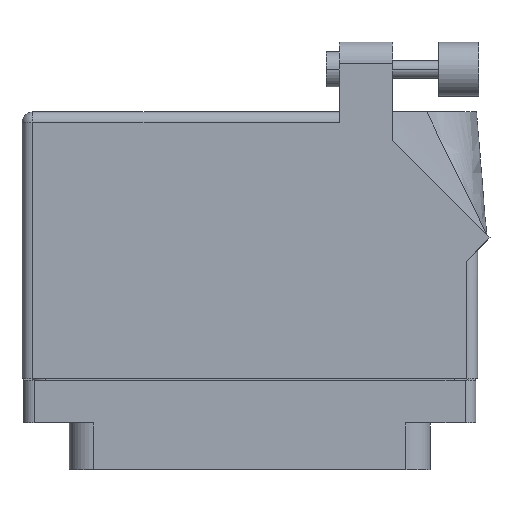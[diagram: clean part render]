
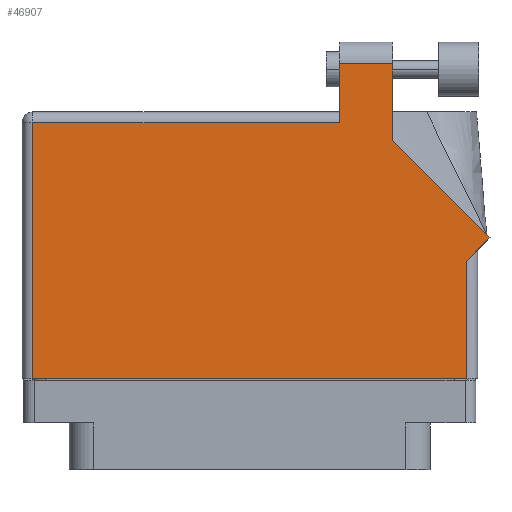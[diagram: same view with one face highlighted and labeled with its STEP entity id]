
A CAD part, front view. The second image highlights one B-rep face of the part: STEP entity #46907.
In plain terms, the highlighted face is planar.
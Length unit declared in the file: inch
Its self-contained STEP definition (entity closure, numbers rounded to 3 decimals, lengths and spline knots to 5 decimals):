
#619 = CARTESIAN_POINT ( 'NONE',  ( -1.306, 1.43, 0.455 ) ) ;
#1910 = ORIENTED_EDGE ( 'NONE', *, *, #14953, .T. ) ;
#3259 = EDGE_LOOP ( 'NONE', ( #28882, #19942, #36924, #26401, #10482, #31854, #46500, #20059, #1910 ) ) ;
#4054 = CARTESIAN_POINT ( 'NONE',  ( -1.306, 1.368, 0.455 ) ) ;
#4148 = FACE_OUTER_BOUND ( 'NONE', #3259, .T. ) ;
#4621 = LINE ( 'NONE', #43150, #7143 ) ;
#6073 = EDGE_CURVE ( 'NONE', #32057, #24403, #44355, .T. ) ;
#6397 = VECTOR ( 'NONE', #47494, 39.37008 ) ;
#7143 = VECTOR ( 'NONE', #19207, 39.37008 ) ;
#7683 = LINE ( 'NONE', #45672, #38993 ) ;
#8617 = VECTOR ( 'NONE', #9817, 39.37008 ) ;
#9040 = DIRECTION ( 'NONE',  ( 0., 0., -1. ) ) ;
#9306 = CARTESIAN_POINT ( 'NONE',  ( 1.37671, 0.70771, 0.455 ) ) ;
#9817 = DIRECTION ( 'NONE',  ( -0.707, 0.707, 0. ) ) ;
#10092 = VERTEX_POINT ( 'NONE', #9306 ) ;
#10482 = ORIENTED_EDGE ( 'NONE', *, *, #15534, .T. ) ;
#10491 = VECTOR ( 'NONE', #27867, 39.37008 ) ;
#10498 = VECTOR ( 'NONE', #36122, 39.37008 ) ;
#13023 = EDGE_CURVE ( 'NONE', #18668, #38605, #38357, .T. ) ;
#13599 = VERTEX_POINT ( 'NONE', #32196 ) ;
#14877 = LINE ( 'NONE', #44491, #10491 ) ;
#14953 = EDGE_CURVE ( 'NONE', #10092, #40217, #46825, .T. ) ;
#15534 = EDGE_CURVE ( 'NONE', #24403, #18668, #25461, .T. ) ;
#18668 = VERTEX_POINT ( 'NONE', #19791 ) ;
#19162 = VERTEX_POINT ( 'NONE', #19208 ) ;
#19207 = DIRECTION ( 'NONE',  ( 0., -1., 0. ) ) ;
#19208 = CARTESIAN_POINT ( 'NONE',  ( 0.513, 1.705, 0.455 ) ) ;
#19791 = CARTESIAN_POINT ( 'NONE',  ( -1.244, -0.1, 0.455 ) ) ;
#19942 = ORIENTED_EDGE ( 'NONE', *, *, #36647, .T. ) ;
#20059 = ORIENTED_EDGE ( 'NONE', *, *, #33033, .T. ) ;
#20361 = CARTESIAN_POINT ( 'NONE',  ( 0.82, 1.26442, 0.455 ) ) ;
#21722 = DIRECTION ( 'NONE',  ( 0.707, 0.707, 0. ) ) ;
#23365 = CARTESIAN_POINT ( 'NONE',  ( -1.306, -0.1, 0.455 ) ) ;
#24403 = VERTEX_POINT ( 'NONE', #25230 ) ;
#24527 = DIRECTION ( 'NONE',  ( 0., 1., 0. ) ) ;
#25230 = CARTESIAN_POINT ( 'NONE',  ( -1.244, 1.368, 0.455 ) ) ;
#25325 = EDGE_CURVE ( 'NONE', #38605, #26138, #28949, .T. ) ;
#25408 = CARTESIAN_POINT ( 'NONE',  ( 0.513, 1.368, 0.455 ) ) ;
#25461 = LINE ( 'NONE', #26735, #32988 ) ;
#26138 = VERTEX_POINT ( 'NONE', #33226 ) ;
#26401 = ORIENTED_EDGE ( 'NONE', *, *, #6073, .T. ) ;
#26735 = CARTESIAN_POINT ( 'NONE',  ( -1.244, -0.1, 0.455 ) ) ;
#27249 = EDGE_CURVE ( 'NONE', #40217, #13599, #30662, .T. ) ;
#27601 = DIRECTION ( 'NONE',  ( 0., 1., 0. ) ) ;
#27867 = DIRECTION ( 'NONE',  ( -1., 0., 0. ) ) ;
#28882 = ORIENTED_EDGE ( 'NONE', *, *, #27249, .T. ) ;
#28949 = LINE ( 'NONE', #51566, #40840 ) ;
#29771 = CARTESIAN_POINT ( 'NONE',  ( 1.37671, 0.70771, 0.455 ) ) ;
#30218 = CARTESIAN_POINT ( 'NONE',  ( 0.82, 1.26442, 0.455 ) ) ;
#30662 = LINE ( 'NONE', #20361, #41294 ) ;
#31854 = ORIENTED_EDGE ( 'NONE', *, *, #13023, .T. ) ;
#32057 = VERTEX_POINT ( 'NONE', #25408 ) ;
#32196 = CARTESIAN_POINT ( 'NONE',  ( 0.82, 1.705, 0.455 ) ) ;
#32224 = EDGE_CURVE ( 'NONE', #19162, #32057, #4621, .T. ) ;
#32964 = AXIS2_PLACEMENT_3D ( 'NONE', #619, #9040, #37049 ) ;
#32988 = VECTOR ( 'NONE', #38104, 39.37008 ) ;
#33033 = EDGE_CURVE ( 'NONE', #26138, #10092, #7683, .T. ) ;
#33226 = CARTESIAN_POINT ( 'NONE',  ( 1.244, 0.575, 0.455 ) ) ;
#36122 = DIRECTION ( 'NONE',  ( -1., 0., 0. ) ) ;
#36647 = EDGE_CURVE ( 'NONE', #13599, #19162, #14877, .T. ) ;
#36924 = ORIENTED_EDGE ( 'NONE', *, *, #32224, .T. ) ;
#37049 = DIRECTION ( 'NONE',  ( -1., 0., 0. ) ) ;
#38104 = DIRECTION ( 'NONE',  ( 0., -1., 0. ) ) ;
#38357 = LINE ( 'NONE', #23365, #6397 ) ;
#38605 = VERTEX_POINT ( 'NONE', #42043 ) ;
#38993 = VECTOR ( 'NONE', #21722, 39.37008 ) ;
#40217 = VERTEX_POINT ( 'NONE', #30218 ) ;
#40840 = VECTOR ( 'NONE', #27601, 39.37008 ) ;
#41294 = VECTOR ( 'NONE', #24527, 39.37008 ) ;
#42043 = CARTESIAN_POINT ( 'NONE',  ( 1.244, -0.1, 0.455 ) ) ;
#43150 = CARTESIAN_POINT ( 'NONE',  ( 0.513, 1.43, 0.455 ) ) ;
#44355 = LINE ( 'NONE', #4054, #10498 ) ;
#44491 = CARTESIAN_POINT ( 'NONE',  ( 0.513, 1.705, 0.455 ) ) ;
#45100 = PLANE ( 'NONE',  #32964 ) ;
#45672 = CARTESIAN_POINT ( 'NONE',  ( 1.306, 0.637, 0.455 ) ) ;
#46500 = ORIENTED_EDGE ( 'NONE', *, *, #25325, .T. ) ;
#46825 = LINE ( 'NONE', #29771, #8617 ) ;
#46907 = ADVANCED_FACE ( 'NONE', ( #4148 ), #45100, .F. ) ;
#47494 = DIRECTION ( 'NONE',  ( 1., 0., 0. ) ) ;
#51566 = CARTESIAN_POINT ( 'NONE',  ( 1.244, 0.637, 0.455 ) ) ;
